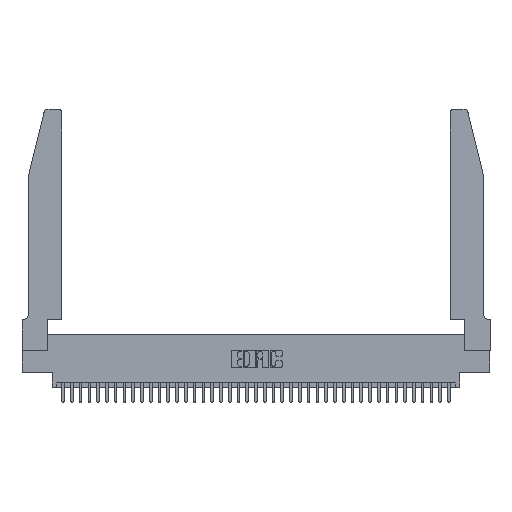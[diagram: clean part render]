
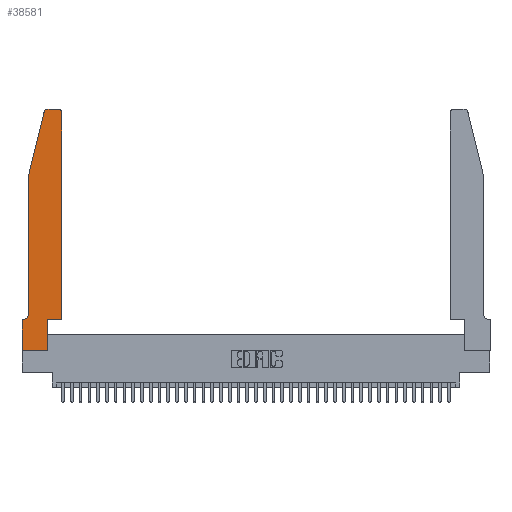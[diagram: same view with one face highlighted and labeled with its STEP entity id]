
A CAD part, top view. The second image highlights one B-rep face of the part: STEP entity #38581.
In plain terms, the highlighted planar face has unit normal (0, 0, 1).
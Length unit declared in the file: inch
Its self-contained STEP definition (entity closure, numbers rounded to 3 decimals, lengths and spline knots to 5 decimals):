
#524 = CARTESIAN_POINT ( 'NONE',  ( 0.0055, 0.42, 0.37 ) ) ;
#795 = LINE ( 'NONE', #4461, #6568 ) ;
#896 = LINE ( 'NONE', #20456, #8106 ) ;
#1142 = CARTESIAN_POINT ( 'NONE',  ( 0., 0., 0.37 ) ) ;
#2672 = CARTESIAN_POINT ( 'NONE',  ( 0., 0., 0.37 ) ) ;
#3383 = DIRECTION ( 'NONE',  ( 0., -1., 0. ) ) ;
#3534 = VECTOR ( 'NONE', #20748, 39.37008 ) ;
#3633 = VERTEX_POINT ( 'NONE', #23140 ) ;
#3779 = LINE ( 'NONE', #13443, #12922 ) ;
#4018 = EDGE_CURVE ( 'NONE', #34602, #18165, #23520, .T. ) ;
#4181 = ORIENTED_EDGE ( 'NONE', *, *, #13276, .T. ) ;
#4461 = CARTESIAN_POINT ( 'NONE',  ( 0.2865, 0.35, 0.37 ) ) ;
#4790 = EDGE_CURVE ( 'NONE', #34190, #5253, #29215, .T. ) ;
#5253 = VERTEX_POINT ( 'NONE', #19307 ) ;
#5524 = DIRECTION ( 'NONE',  ( 0., 0., 1. ) ) ;
#5816 = ORIENTED_EDGE ( 'NONE', *, *, #24782, .T. ) ;
#6272 = EDGE_CURVE ( 'NONE', #18654, #23033, #6424, .T. ) ;
#6340 = CARTESIAN_POINT ( 'NONE',  ( 0.0055, 0.35, 0.37 ) ) ;
#6424 = LINE ( 'NONE', #26812, #3534 ) ;
#6568 = VECTOR ( 'NONE', #7266, 39.37008 ) ;
#6839 = VERTEX_POINT ( 'NONE', #13906 ) ;
#7184 = DIRECTION ( 'NONE',  ( 0., -1., 0. ) ) ;
#7266 = DIRECTION ( 'NONE',  ( 0., 1., 0. ) ) ;
#7708 = CARTESIAN_POINT ( 'NONE',  ( 0.2865, 0., 0.37 ) ) ;
#8106 = VECTOR ( 'NONE', #38916, 39.37008 ) ;
#8361 = CARTESIAN_POINT ( 'NONE',  ( 0.4505, 0.35, 0.37 ) ) ;
#9253 = DIRECTION ( 'NONE',  ( 0., 1., 0. ) ) ;
#10142 = AXIS2_PLACEMENT_3D ( 'NONE', #524, #18852, #28001 ) ;
#10993 = EDGE_CURVE ( 'NONE', #34907, #3633, #18395, .T. ) ;
#11678 = DIRECTION ( 'NONE',  ( 0., 0., 1. ) ) ;
#11894 = LINE ( 'NONE', #1142, #37919 ) ;
#12186 = CARTESIAN_POINT ( 'NONE',  ( 0., 0.35, 0.37 ) ) ;
#12870 = CARTESIAN_POINT ( 'NONE',  ( 0.4505, 0.35, 0.37 ) ) ;
#12922 = VECTOR ( 'NONE', #38542, 39.37008 ) ;
#12935 = CARTESIAN_POINT ( 'NONE',  ( 0.4505, 2.72, 0.37 ) ) ;
#13276 = EDGE_CURVE ( 'NONE', #15796, #35274, #32260, .T. ) ;
#13443 = CARTESIAN_POINT ( 'NONE',  ( 0.0755, 2., 0.37 ) ) ;
#13906 = CARTESIAN_POINT ( 'NONE',  ( 0.0755, 0.42, 0.37 ) ) ;
#13924 = ORIENTED_EDGE ( 'NONE', *, *, #4018, .T. ) ;
#14161 = EDGE_CURVE ( 'NONE', #23033, #34602, #11894, .T. ) ;
#14190 = ORIENTED_EDGE ( 'NONE', *, *, #10993, .T. ) ;
#14290 = ORIENTED_EDGE ( 'NONE', *, *, #20531, .T. ) ;
#14780 = ORIENTED_EDGE ( 'NONE', *, *, #4790, .T. ) ;
#14810 = DIRECTION ( 'NONE',  ( 1., 0., 0. ) ) ;
#15635 = ORIENTED_EDGE ( 'NONE', *, *, #18753, .T. ) ;
#15796 = VERTEX_POINT ( 'NONE', #12935 ) ;
#16048 = EDGE_CURVE ( 'NONE', #5253, #15796, #23834, .T. ) ;
#17358 = EDGE_CURVE ( 'NONE', #6839, #18654, #33806, .T. ) ;
#17649 = VECTOR ( 'NONE', #25560, 39.37008 ) ;
#17653 = VECTOR ( 'NONE', #21541, 39.37008 ) ;
#17654 = ORIENTED_EDGE ( 'NONE', *, *, #14161, .T. ) ;
#18165 = VERTEX_POINT ( 'NONE', #7708 ) ;
#18395 = CIRCLE ( 'NONE', #18551, 0.03 ) ;
#18551 = AXIS2_PLACEMENT_3D ( 'NONE', #30145, #11678, #24268 ) ;
#18654 = VERTEX_POINT ( 'NONE', #6340 ) ;
#18695 = EDGE_CURVE ( 'NONE', #3633, #28326, #3779, .T. ) ;
#18753 = EDGE_CURVE ( 'NONE', #35274, #34907, #896, .T. ) ;
#18852 = DIRECTION ( 'NONE',  ( 0., 0., -1. ) ) ;
#19307 = CARTESIAN_POINT ( 'NONE',  ( 0.4505, 0.35, 0.37 ) ) ;
#20257 = ORIENTED_EDGE ( 'NONE', *, *, #17358, .T. ) ;
#20456 = CARTESIAN_POINT ( 'NONE',  ( 0.2605, 2.75, 0.37 ) ) ;
#20531 = EDGE_CURVE ( 'NONE', #18165, #34190, #795, .T. ) ;
#20748 = DIRECTION ( 'NONE',  ( -1., 0., 0. ) ) ;
#21541 = DIRECTION ( 'NONE',  ( 1., 0., 0. ) ) ;
#22511 = VECTOR ( 'NONE', #3383, 39.37008 ) ;
#22770 = AXIS2_PLACEMENT_3D ( 'NONE', #33429, #5524, #14810 ) ;
#23033 = VERTEX_POINT ( 'NONE', #12186 ) ;
#23140 = CARTESIAN_POINT ( 'NONE',  ( 0.25487, 2.72718, 0.37 ) ) ;
#23361 = EDGE_LOOP ( 'NONE', ( #15635, #14190, #23947, #5816, #20257, #38422, #17654, #13924, #14290, #14780, #30558, #4181 ) ) ;
#23520 = LINE ( 'NONE', #36781, #17649 ) ;
#23834 = LINE ( 'NONE', #12870, #36302 ) ;
#23947 = ORIENTED_EDGE ( 'NONE', *, *, #18695, .T. ) ;
#24268 = DIRECTION ( 'NONE',  ( 1., 0., 0. ) ) ;
#24384 = DIRECTION ( 'NONE',  ( 0., 0., 1. ) ) ;
#24782 = EDGE_CURVE ( 'NONE', #28326, #6839, #32572, .T. ) ;
#25560 = DIRECTION ( 'NONE',  ( 1., 0., 0. ) ) ;
#26812 = CARTESIAN_POINT ( 'NONE',  ( 0.0755, 0.35, 0.37 ) ) ;
#27467 = CARTESIAN_POINT ( 'NONE',  ( 0.2865, 0.35, 0.37 ) ) ;
#27897 = CARTESIAN_POINT ( 'NONE',  ( 0.0755, 2., 0.37 ) ) ;
#28001 = DIRECTION ( 'NONE',  ( -1., 0., 0. ) ) ;
#28326 = VERTEX_POINT ( 'NONE', #32731 ) ;
#29215 = LINE ( 'NONE', #8361, #17653 ) ;
#29811 = CARTESIAN_POINT ( 'NONE',  ( 0.4205, 2.75, 0.37 ) ) ;
#30145 = CARTESIAN_POINT ( 'NONE',  ( 0.284, 2.72, 0.37 ) ) ;
#30541 = PLANE ( 'NONE',  #34231 ) ;
#30558 = ORIENTED_EDGE ( 'NONE', *, *, #16048, .T. ) ;
#31709 = CARTESIAN_POINT ( 'NONE',  ( 0.284, 2.75, 0.37 ) ) ;
#32260 = CIRCLE ( 'NONE', #22770, 0.03 ) ;
#32572 = LINE ( 'NONE', #27897, #22511 ) ;
#32731 = CARTESIAN_POINT ( 'NONE',  ( 0.0755, 2., 0.37 ) ) ;
#33429 = CARTESIAN_POINT ( 'NONE',  ( 0.4205, 2.72, 0.37 ) ) ;
#33498 = DIRECTION ( 'NONE',  ( 1., 0., 0. ) ) ;
#33806 = CIRCLE ( 'NONE', #10142, 0.07 ) ;
#34190 = VERTEX_POINT ( 'NONE', #27467 ) ;
#34231 = AXIS2_PLACEMENT_3D ( 'NONE', #39299, #24384, #33498 ) ;
#34602 = VERTEX_POINT ( 'NONE', #2672 ) ;
#34907 = VERTEX_POINT ( 'NONE', #31709 ) ;
#35274 = VERTEX_POINT ( 'NONE', #29811 ) ;
#36302 = VECTOR ( 'NONE', #9253, 39.37008 ) ;
#36781 = CARTESIAN_POINT ( 'NONE',  ( 0., 0., 0.37 ) ) ;
#36786 = FACE_OUTER_BOUND ( 'NONE', #23361, .T. ) ;
#37919 = VECTOR ( 'NONE', #7184, 39.37008 ) ;
#38422 = ORIENTED_EDGE ( 'NONE', *, *, #6272, .T. ) ;
#38542 = DIRECTION ( 'NONE',  ( -0.239, -0.971, 0. ) ) ;
#38581 = ADVANCED_FACE ( 'NONE', ( #36786 ), #30541, .T. ) ;
#38916 = DIRECTION ( 'NONE',  ( -1., 0., 0. ) ) ;
#39299 = CARTESIAN_POINT ( 'NONE',  ( 0., 0.35, 0.37 ) ) ;
